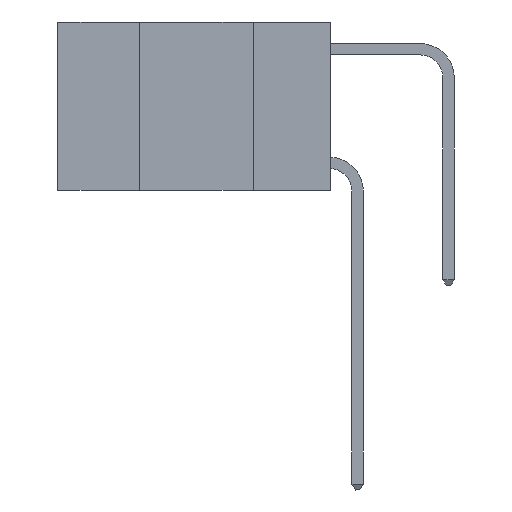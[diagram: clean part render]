
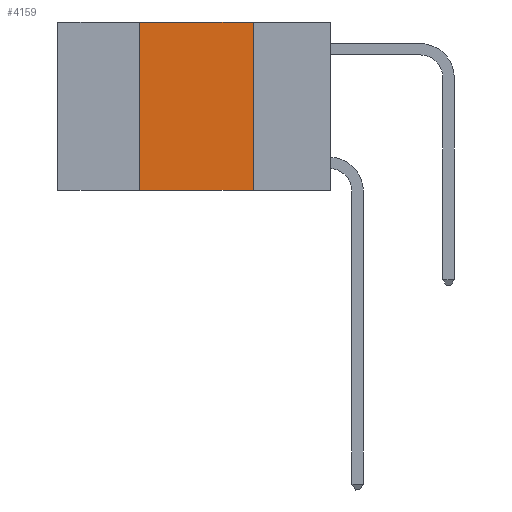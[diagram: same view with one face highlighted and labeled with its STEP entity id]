
A CAD part, left-side view. The second image highlights one B-rep face of the part: STEP entity #4159.
In plain terms, the highlighted planar face has unit normal (-1, 0, 0).
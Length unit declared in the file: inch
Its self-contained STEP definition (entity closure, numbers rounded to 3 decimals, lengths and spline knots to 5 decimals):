
#382 = DIRECTION ( 'NONE',  ( 0., -1., 0. ) ) ;
#1947 = DIRECTION ( 'NONE',  ( 0., 0., 1. ) ) ;
#2080 = EDGE_LOOP ( 'NONE', ( #13524, #15566, #13293, #3084 ) ) ;
#2174 = CARTESIAN_POINT ( 'NONE',  ( 0., 0.42, -0.37 ) ) ;
#2428 = VECTOR ( 'NONE', #382, 39.37008 ) ;
#3084 = ORIENTED_EDGE ( 'NONE', *, *, #14797, .T. ) ;
#3802 = VERTEX_POINT ( 'NONE', #8066 ) ;
#3874 = EDGE_CURVE ( 'NONE', #3802, #12680, #6831, .T. ) ;
#4159 = ADVANCED_FACE ( 'NONE', ( #14501 ), #6348, .F. ) ;
#4421 = VERTEX_POINT ( 'NONE', #6077 ) ;
#4636 = LINE ( 'NONE', #6058, #17367 ) ;
#5117 = EDGE_CURVE ( 'NONE', #4421, #3802, #12653, .T. ) ;
#5635 = DIRECTION ( 'NONE',  ( 0., -1., 0. ) ) ;
#6058 = CARTESIAN_POINT ( 'NONE',  ( 0., 0.42, 0. ) ) ;
#6076 = EDGE_CURVE ( 'NONE', #9400, #4421, #4636, .T. ) ;
#6077 = CARTESIAN_POINT ( 'NONE',  ( 0., 0.42, 0. ) ) ;
#6348 = PLANE ( 'NONE',  #7408 ) ;
#6831 = LINE ( 'NONE', #13640, #17156 ) ;
#7408 = AXIS2_PLACEMENT_3D ( 'NONE', #14771, #17379, #10608 ) ;
#7450 = CARTESIAN_POINT ( 'NONE',  ( 0., 0.17, -0.37 ) ) ;
#8066 = CARTESIAN_POINT ( 'NONE',  ( 0., 0.17, 0. ) ) ;
#8334 = CARTESIAN_POINT ( 'NONE',  ( 0., 0.6, 0. ) ) ;
#9400 = VERTEX_POINT ( 'NONE', #2174 ) ;
#9612 = VECTOR ( 'NONE', #5635, 39.37008 ) ;
#10608 = DIRECTION ( 'NONE',  ( 0., 0., -1. ) ) ;
#10871 = CARTESIAN_POINT ( 'NONE',  ( 0., 0.6, -0.37 ) ) ;
#12194 = LINE ( 'NONE', #10871, #9612 ) ;
#12653 = LINE ( 'NONE', #8334, #2428 ) ;
#12680 = VERTEX_POINT ( 'NONE', #7450 ) ;
#13293 = ORIENTED_EDGE ( 'NONE', *, *, #6076, .F. ) ;
#13524 = ORIENTED_EDGE ( 'NONE', *, *, #3874, .F. ) ;
#13640 = CARTESIAN_POINT ( 'NONE',  ( 0., 0.17, 0. ) ) ;
#14501 = FACE_OUTER_BOUND ( 'NONE', #2080, .T. ) ;
#14771 = CARTESIAN_POINT ( 'NONE',  ( 0., 0.6, 0. ) ) ;
#14797 = EDGE_CURVE ( 'NONE', #9400, #12680, #12194, .T. ) ;
#15061 = DIRECTION ( 'NONE',  ( 0., 0., -1. ) ) ;
#15566 = ORIENTED_EDGE ( 'NONE', *, *, #5117, .F. ) ;
#17156 = VECTOR ( 'NONE', #15061, 39.37008 ) ;
#17367 = VECTOR ( 'NONE', #1947, 39.37008 ) ;
#17379 = DIRECTION ( 'NONE',  ( 1., 0., 0. ) ) ;
